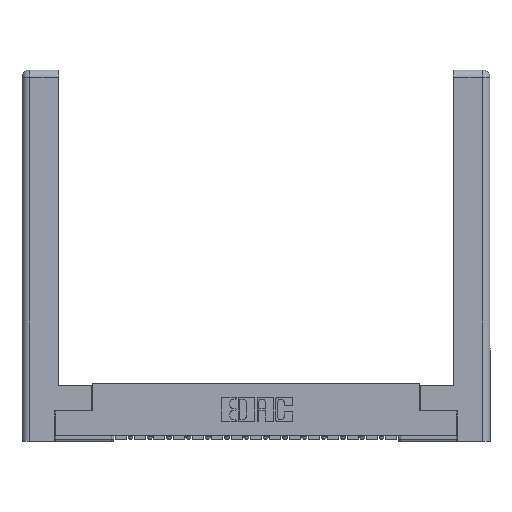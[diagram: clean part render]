
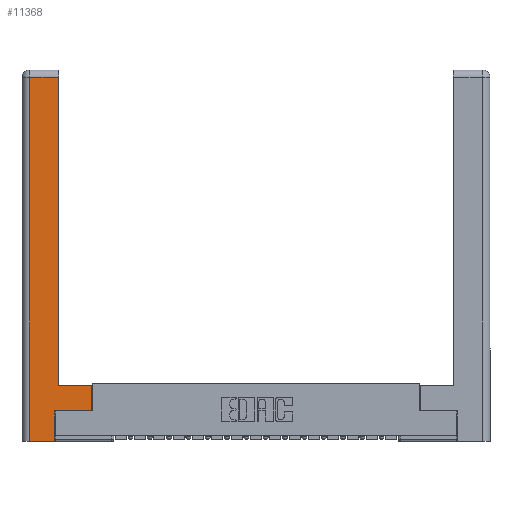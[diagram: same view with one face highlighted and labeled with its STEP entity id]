
A CAD part, top view. The second image highlights one B-rep face of the part: STEP entity #11368.
In plain terms, the highlighted planar face has unit normal (0, 0, 1).
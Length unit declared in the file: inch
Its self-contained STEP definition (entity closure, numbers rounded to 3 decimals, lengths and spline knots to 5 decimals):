
#1251 = VERTEX_POINT ( 'NONE', #17141 ) ;
#1284 = EDGE_CURVE ( 'NONE', #8000, #5106, #3460, .T. ) ;
#1661 = EDGE_CURVE ( 'NONE', #13499, #8000, #10112, .T. ) ;
#1808 = VECTOR ( 'NONE', #9643, 39.37008 ) ;
#1947 = VERTEX_POINT ( 'NONE', #10465 ) ;
#2211 = VECTOR ( 'NONE', #11920, 39.37008 ) ;
#2630 = CARTESIAN_POINT ( 'NONE',  ( 0.295, 2.94, 0. ) ) ;
#2930 = LINE ( 'NONE', #5919, #2211 ) ;
#3072 = VERTEX_POINT ( 'NONE', #12852 ) ;
#3460 = LINE ( 'NONE', #6393, #1808 ) ;
#3466 = ORIENTED_EDGE ( 'NONE', *, *, #1284, .T. ) ;
#3924 = DIRECTION ( 'NONE',  ( 0., 0., -1. ) ) ;
#4080 = ORIENTED_EDGE ( 'NONE', *, *, #7240, .T. ) ;
#4416 = CARTESIAN_POINT ( 'NONE',  ( 0.265, 0.245, 0. ) ) ;
#5106 = VERTEX_POINT ( 'NONE', #2630 ) ;
#5211 = ORIENTED_EDGE ( 'NONE', *, *, #17587, .T. ) ;
#5391 = DIRECTION ( 'NONE',  ( 0., 1., 0. ) ) ;
#5507 = CARTESIAN_POINT ( 'NONE',  ( 0.0615, 2.94, 0. ) ) ;
#5919 = CARTESIAN_POINT ( 'NONE',  ( 0.265, 0., 0. ) ) ;
#6393 = CARTESIAN_POINT ( 'NONE',  ( 0.295, 3., 0. ) ) ;
#6401 = CARTESIAN_POINT ( 'NONE',  ( 0.0615, 0., 0. ) ) ;
#6447 = CARTESIAN_POINT ( 'NONE',  ( 0.265, 0.245, 0. ) ) ;
#6502 = ORIENTED_EDGE ( 'NONE', *, *, #13575, .T. ) ;
#7135 = DIRECTION ( 'NONE',  ( 1., 0., 0. ) ) ;
#7240 = EDGE_CURVE ( 'NONE', #1947, #3072, #13067, .T. ) ;
#7338 = EDGE_LOOP ( 'NONE', ( #3466, #7851, #4080, #17084, #5211, #6502, #18403, #19586 ) ) ;
#7851 = ORIENTED_EDGE ( 'NONE', *, *, #10132, .T. ) ;
#8000 = VERTEX_POINT ( 'NONE', #12464 ) ;
#9188 = VECTOR ( 'NONE', #16130, 39.37008 ) ;
#9464 = VECTOR ( 'NONE', #5391, 39.37008 ) ;
#9643 = DIRECTION ( 'NONE',  ( 0., 1., 0. ) ) ;
#10063 = CARTESIAN_POINT ( 'NONE',  ( 0.565, 0.245, 0. ) ) ;
#10112 = LINE ( 'NONE', #10756, #10805 ) ;
#10132 = EDGE_CURVE ( 'NONE', #5106, #1947, #19469, .T. ) ;
#10465 = CARTESIAN_POINT ( 'NONE',  ( 0.0615, 2.94, 0. ) ) ;
#10756 = CARTESIAN_POINT ( 'NONE',  ( 0.295, 0.45, 0. ) ) ;
#10805 = VECTOR ( 'NONE', #15186, 39.37008 ) ;
#11368 = ADVANCED_FACE ( 'NONE', ( #17744 ), #19212, .F. ) ;
#11397 = CARTESIAN_POINT ( 'NONE',  ( 0.565, 0.45, 0. ) ) ;
#11445 = AXIS2_PLACEMENT_3D ( 'NONE', #14676, #3924, #19348 ) ;
#11596 = EDGE_CURVE ( 'NONE', #3072, #1251, #2930, .T. ) ;
#11920 = DIRECTION ( 'NONE',  ( 1., 0., 0. ) ) ;
#12409 = VECTOR ( 'NONE', #7135, 39.37008 ) ;
#12464 = CARTESIAN_POINT ( 'NONE',  ( 0.295, 0.45, 0. ) ) ;
#12852 = CARTESIAN_POINT ( 'NONE',  ( 0.0615, 0., 0. ) ) ;
#13067 = LINE ( 'NONE', #6401, #13791 ) ;
#13158 = CARTESIAN_POINT ( 'NONE',  ( 0.565, 0.245, 0. ) ) ;
#13499 = VERTEX_POINT ( 'NONE', #15697 ) ;
#13531 = VERTEX_POINT ( 'NONE', #13158 ) ;
#13575 = EDGE_CURVE ( 'NONE', #19211, #13531, #13850, .T. ) ;
#13791 = VECTOR ( 'NONE', #13894, 39.37008 ) ;
#13850 = LINE ( 'NONE', #10063, #12409 ) ;
#13894 = DIRECTION ( 'NONE',  ( 0., -1., 0. ) ) ;
#13998 = DIRECTION ( 'NONE',  ( 0., 1., 0. ) ) ;
#14676 = CARTESIAN_POINT ( 'NONE',  ( 0., 0., 0. ) ) ;
#15186 = DIRECTION ( 'NONE',  ( -1., 0., 0. ) ) ;
#15445 = LINE ( 'NONE', #6447, #19504 ) ;
#15697 = CARTESIAN_POINT ( 'NONE',  ( 0.565, 0.45, 0. ) ) ;
#16130 = DIRECTION ( 'NONE',  ( -1., 0., 0. ) ) ;
#17084 = ORIENTED_EDGE ( 'NONE', *, *, #11596, .T. ) ;
#17141 = CARTESIAN_POINT ( 'NONE',  ( 0.265, 0., 0. ) ) ;
#17240 = EDGE_CURVE ( 'NONE', #13531, #13499, #19523, .T. ) ;
#17587 = EDGE_CURVE ( 'NONE', #1251, #19211, #15445, .T. ) ;
#17744 = FACE_OUTER_BOUND ( 'NONE', #7338, .T. ) ;
#18403 = ORIENTED_EDGE ( 'NONE', *, *, #17240, .T. ) ;
#19211 = VERTEX_POINT ( 'NONE', #4416 ) ;
#19212 = PLANE ( 'NONE',  #11445 ) ;
#19348 = DIRECTION ( 'NONE',  ( -1., 0., 0. ) ) ;
#19469 = LINE ( 'NONE', #5507, #9188 ) ;
#19504 = VECTOR ( 'NONE', #13998, 39.37008 ) ;
#19523 = LINE ( 'NONE', #11397, #9464 ) ;
#19586 = ORIENTED_EDGE ( 'NONE', *, *, #1661, .T. ) ;
